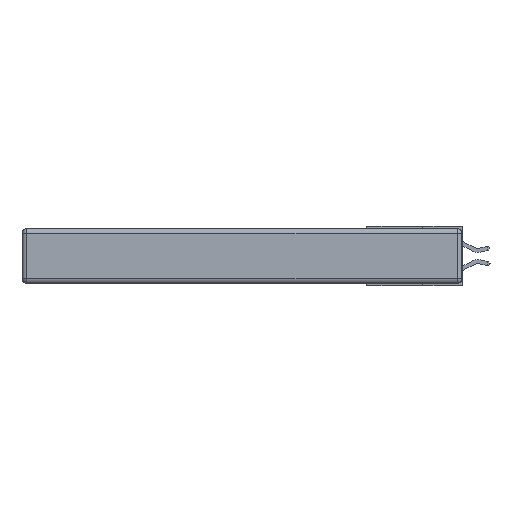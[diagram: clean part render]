
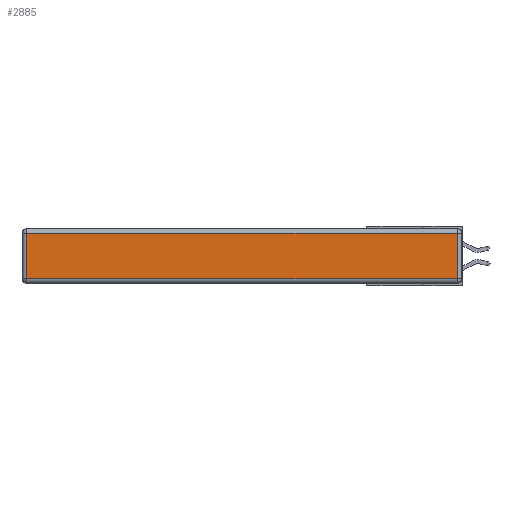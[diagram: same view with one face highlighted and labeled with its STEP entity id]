
A CAD part, left-side view. The second image highlights one B-rep face of the part: STEP entity #2885.
In plain terms, the highlighted planar face has unit normal (-1, 0, 0).
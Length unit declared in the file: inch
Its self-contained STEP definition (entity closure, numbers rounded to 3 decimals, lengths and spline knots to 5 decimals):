
#204 = ORIENTED_EDGE ( 'NONE', *, *, #657, .T. ) ;
#434 = DIRECTION ( 'NONE',  ( 0., 1., 0. ) ) ;
#545 = VERTEX_POINT ( 'NONE', #23960 ) ;
#657 = EDGE_CURVE ( 'NONE', #16729, #545, #30859, .T. ) ;
#1884 = EDGE_CURVE ( 'NONE', #545, #21493, #13186, .T. ) ;
#2539 = CARTESIAN_POINT ( 'NONE',  ( 0., 0.03, -0.03 ) ) ;
#2885 = ADVANCED_FACE ( 'NONE', ( #3954 ), #28464, .T. ) ;
#3954 = FACE_OUTER_BOUND ( 'NONE', #32969, .T. ) ;
#4124 = CARTESIAN_POINT ( 'NONE',  ( 0., 0.03, -0.343 ) ) ;
#4226 = DIRECTION ( 'NONE',  ( 0., 0., 1. ) ) ;
#4378 = VECTOR ( 'NONE', #434, 39.37008 ) ;
#4733 = AXIS2_PLACEMENT_3D ( 'NONE', #23395, #23175, #15624 ) ;
#4980 = CARTESIAN_POINT ( 'NONE',  ( 0., 2.75, -0.03 ) ) ;
#5211 = VECTOR ( 'NONE', #4226, 39.37008 ) ;
#6697 = LINE ( 'NONE', #25895, #14693 ) ;
#8173 = DIRECTION ( 'NONE',  ( 0., 0., -1. ) ) ;
#9447 = EDGE_CURVE ( 'NONE', #21493, #9992, #21505, .T. ) ;
#9992 = VERTEX_POINT ( 'NONE', #24220 ) ;
#11134 = ORIENTED_EDGE ( 'NONE', *, *, #31604, .T. ) ;
#13186 = LINE ( 'NONE', #4124, #5211 ) ;
#13446 = CARTESIAN_POINT ( 'NONE',  ( 0., 2.72, -0.313 ) ) ;
#14047 = DIRECTION ( 'NONE',  ( 0., -1., 0. ) ) ;
#14693 = VECTOR ( 'NONE', #8173, 39.37008 ) ;
#15624 = DIRECTION ( 'NONE',  ( 0., 0., 1. ) ) ;
#16729 = VERTEX_POINT ( 'NONE', #13446 ) ;
#21493 = VERTEX_POINT ( 'NONE', #2539 ) ;
#21505 = LINE ( 'NONE', #4980, #4378 ) ;
#21514 = ORIENTED_EDGE ( 'NONE', *, *, #9447, .T. ) ;
#21728 = CARTESIAN_POINT ( 'NONE',  ( 0., 0., -0.313 ) ) ;
#23175 = DIRECTION ( 'NONE',  ( -1., 0., 0. ) ) ;
#23395 = CARTESIAN_POINT ( 'NONE',  ( 0., 0., -0.343 ) ) ;
#23960 = CARTESIAN_POINT ( 'NONE',  ( 0., 0.03, -0.313 ) ) ;
#24062 = VECTOR ( 'NONE', #14047, 39.37008 ) ;
#24190 = ORIENTED_EDGE ( 'NONE', *, *, #1884, .T. ) ;
#24220 = CARTESIAN_POINT ( 'NONE',  ( 0., 2.72, -0.03 ) ) ;
#25895 = CARTESIAN_POINT ( 'NONE',  ( 0., 2.72, -0.343 ) ) ;
#28464 = PLANE ( 'NONE',  #4733 ) ;
#30859 = LINE ( 'NONE', #21728, #24062 ) ;
#31604 = EDGE_CURVE ( 'NONE', #9992, #16729, #6697, .T. ) ;
#32969 = EDGE_LOOP ( 'NONE', ( #204, #24190, #21514, #11134 ) ) ;
